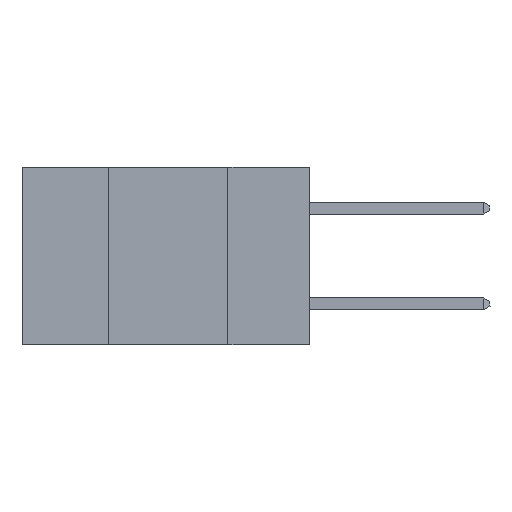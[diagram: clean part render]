
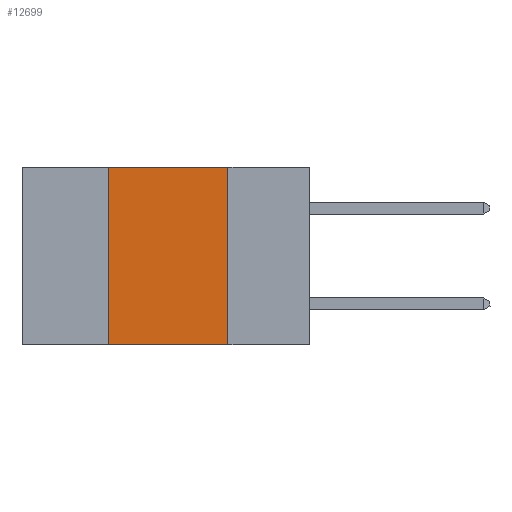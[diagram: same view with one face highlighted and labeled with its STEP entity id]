
A CAD part, left-side view. The second image highlights one B-rep face of the part: STEP entity #12699.
In plain terms, the highlighted planar face has unit normal (-1, 0, 0).
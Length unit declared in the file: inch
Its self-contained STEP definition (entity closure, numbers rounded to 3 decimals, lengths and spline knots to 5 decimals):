
#465 = AXIS2_PLACEMENT_3D ( 'NONE', #14504, #14267, #15624 ) ;
#1196 = DIRECTION ( 'NONE',  ( 0., -1., 0. ) ) ;
#1313 = VECTOR ( 'NONE', #1196, 39.37008 ) ;
#3061 = CARTESIAN_POINT ( 'NONE',  ( 0., 0.42, 0. ) ) ;
#3883 = DIRECTION ( 'NONE',  ( 0., -1., 0. ) ) ;
#4594 = CARTESIAN_POINT ( 'NONE',  ( 0., 0.17, 0. ) ) ;
#4685 = ORIENTED_EDGE ( 'NONE', *, *, #12326, .F. ) ;
#4811 = PLANE ( 'NONE',  #465 ) ;
#5092 = VECTOR ( 'NONE', #16754, 39.37008 ) ;
#5489 = ORIENTED_EDGE ( 'NONE', *, *, #9632, .F. ) ;
#5660 = EDGE_CURVE ( 'NONE', #16749, #12949, #9668, .T. ) ;
#9300 = FACE_OUTER_BOUND ( 'NONE', #17193, .T. ) ;
#9632 = EDGE_CURVE ( 'NONE', #12949, #15734, #14843, .T. ) ;
#9668 = LINE ( 'NONE', #3061, #16221 ) ;
#9843 = CARTESIAN_POINT ( 'NONE',  ( 0., 0.17, -0.37 ) ) ;
#10828 = CARTESIAN_POINT ( 'NONE',  ( 0., 0.6, 0. ) ) ;
#10935 = VERTEX_POINT ( 'NONE', #9843 ) ;
#11458 = LINE ( 'NONE', #4594, #5092 ) ;
#11620 = LINE ( 'NONE', #17290, #16030 ) ;
#12205 = CARTESIAN_POINT ( 'NONE',  ( 0., 0.17, 0. ) ) ;
#12326 = EDGE_CURVE ( 'NONE', #15734, #10935, #11458, .T. ) ;
#12699 = ADVANCED_FACE ( 'NONE', ( #9300 ), #4811, .F. ) ;
#12862 = ORIENTED_EDGE ( 'NONE', *, *, #5660, .F. ) ;
#12949 = VERTEX_POINT ( 'NONE', #14605 ) ;
#13712 = EDGE_CURVE ( 'NONE', #16749, #10935, #11620, .T. ) ;
#14011 = DIRECTION ( 'NONE',  ( 0., 0., 1. ) ) ;
#14124 = ORIENTED_EDGE ( 'NONE', *, *, #13712, .T. ) ;
#14267 = DIRECTION ( 'NONE',  ( 1., 0., 0. ) ) ;
#14504 = CARTESIAN_POINT ( 'NONE',  ( 0., 0.6, 0. ) ) ;
#14605 = CARTESIAN_POINT ( 'NONE',  ( 0., 0.42, 0. ) ) ;
#14843 = LINE ( 'NONE', #10828, #1313 ) ;
#15250 = CARTESIAN_POINT ( 'NONE',  ( 0., 0.42, -0.37 ) ) ;
#15624 = DIRECTION ( 'NONE',  ( 0., 0., -1. ) ) ;
#15734 = VERTEX_POINT ( 'NONE', #12205 ) ;
#16030 = VECTOR ( 'NONE', #3883, 39.37008 ) ;
#16221 = VECTOR ( 'NONE', #14011, 39.37008 ) ;
#16749 = VERTEX_POINT ( 'NONE', #15250 ) ;
#16754 = DIRECTION ( 'NONE',  ( 0., 0., -1. ) ) ;
#17193 = EDGE_LOOP ( 'NONE', ( #4685, #5489, #12862, #14124 ) ) ;
#17290 = CARTESIAN_POINT ( 'NONE',  ( 0., 0.6, -0.37 ) ) ;
